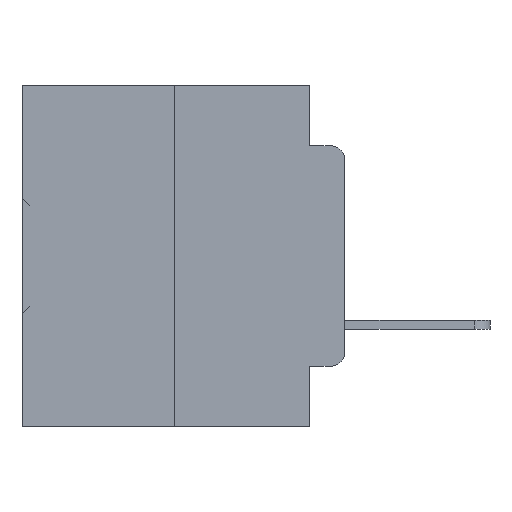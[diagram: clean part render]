
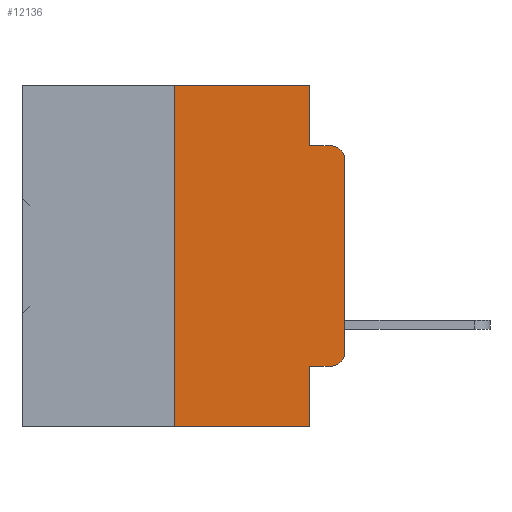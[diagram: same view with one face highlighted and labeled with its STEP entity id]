
A CAD part, left-side view. The second image highlights one B-rep face of the part: STEP entity #12136.
In plain terms, the highlighted planar face has unit normal (-1, 0, 0).
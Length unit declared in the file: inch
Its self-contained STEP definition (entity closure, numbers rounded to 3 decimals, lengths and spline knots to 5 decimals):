
#571 = VECTOR ( 'NONE', #16292, 39.37008 ) ;
#1025 = CARTESIAN_POINT ( 'NONE',  ( 0., 0.051, 0. ) ) ;
#1138 = DIRECTION ( 'NONE',  ( 0., 0., -1. ) ) ;
#1573 = LINE ( 'NONE', #26311, #32571 ) ;
#1580 = LINE ( 'NONE', #21973, #571 ) ;
#2053 = CIRCLE ( 'NONE', #19394, 0.02 ) ;
#2070 = VECTOR ( 'NONE', #13474, 39.37008 ) ;
#2139 = DIRECTION ( 'NONE',  ( 0., -1., 0. ) ) ;
#3630 = PLANE ( 'NONE',  #37530 ) ;
#4343 = EDGE_CURVE ( 'NONE', #12615, #32182, #33869, .T. ) ;
#5000 = CARTESIAN_POINT ( 'NONE',  ( 0., 0.02, -0.1085 ) ) ;
#5078 = VERTEX_POINT ( 'NONE', #11456 ) ;
#5144 = LINE ( 'NONE', #28191, #6150 ) ;
#5808 = CARTESIAN_POINT ( 'NONE',  ( 0., 0.25, 0. ) ) ;
#6150 = VECTOR ( 'NONE', #7257, 39.37008 ) ;
#6776 = CARTESIAN_POINT ( 'NONE',  ( 0., 0., -0.3915 ) ) ;
#6820 = DIRECTION ( 'NONE',  ( 1., 0., 0. ) ) ;
#7229 = VERTEX_POINT ( 'NONE', #32463 ) ;
#7257 = DIRECTION ( 'NONE',  ( 0., 0., -1. ) ) ;
#7376 = VERTEX_POINT ( 'NONE', #6776 ) ;
#7852 = ORIENTED_EDGE ( 'NONE', *, *, #37434, .T. ) ;
#8065 = ORIENTED_EDGE ( 'NONE', *, *, #36766, .T. ) ;
#8166 = DIRECTION ( 'NONE',  ( 0., 0., -1. ) ) ;
#8482 = ORIENTED_EDGE ( 'NONE', *, *, #33053, .F. ) ;
#8788 = ORIENTED_EDGE ( 'NONE', *, *, #32774, .F. ) ;
#9001 = ORIENTED_EDGE ( 'NONE', *, *, #15532, .F. ) ;
#9084 = LINE ( 'NONE', #19105, #24102 ) ;
#9285 = CARTESIAN_POINT ( 'NONE',  ( 0., 0., -0.1085 ) ) ;
#9809 = VECTOR ( 'NONE', #12355, 39.37008 ) ;
#10069 = ORIENTED_EDGE ( 'NONE', *, *, #30841, .F. ) ;
#10225 = ORIENTED_EDGE ( 'NONE', *, *, #4343, .T. ) ;
#11456 = CARTESIAN_POINT ( 'NONE',  ( 0., 0.02, -0.0885 ) ) ;
#11691 = ORIENTED_EDGE ( 'NONE', *, *, #21473, .T. ) ;
#12136 = ADVANCED_FACE ( 'NONE', ( #18305 ), #3630, .F. ) ;
#12290 = ORIENTED_EDGE ( 'NONE', *, *, #24694, .F. ) ;
#12355 = DIRECTION ( 'NONE',  ( 0., 0., 1. ) ) ;
#12615 = VERTEX_POINT ( 'NONE', #27501 ) ;
#13474 = DIRECTION ( 'NONE',  ( 0., -1., 0. ) ) ;
#14044 = CARTESIAN_POINT ( 'NONE',  ( 0., 0.25, 0. ) ) ;
#14267 = DIRECTION ( 'NONE',  ( 0., 0., 1. ) ) ;
#14450 = LINE ( 'NONE', #30665, #20389 ) ;
#15532 = EDGE_CURVE ( 'NONE', #23232, #34252, #14450, .T. ) ;
#16114 = CARTESIAN_POINT ( 'NONE',  ( 0., 0.473, 0. ) ) ;
#16288 = DIRECTION ( 'NONE',  ( 0., -1., 0. ) ) ;
#16292 = DIRECTION ( 'NONE',  ( 0., -1., 0. ) ) ;
#16732 = VERTEX_POINT ( 'NONE', #30584 ) ;
#17167 = LINE ( 'NONE', #37099, #31552 ) ;
#17635 = VERTEX_POINT ( 'NONE', #33755 ) ;
#18305 = FACE_OUTER_BOUND ( 'NONE', #27579, .T. ) ;
#18633 = CIRCLE ( 'NONE', #28339, 0.02 ) ;
#19105 = CARTESIAN_POINT ( 'NONE',  ( 0., 0.051, 0. ) ) ;
#19248 = ORIENTED_EDGE ( 'NONE', *, *, #21204, .T. ) ;
#19394 = AXIS2_PLACEMENT_3D ( 'NONE', #5000, #26105, #8166 ) ;
#19705 = DIRECTION ( 'NONE',  ( -1., 0., 0. ) ) ;
#20389 = VECTOR ( 'NONE', #16288, 39.37008 ) ;
#21204 = EDGE_CURVE ( 'NONE', #7229, #7376, #18633, .T. ) ;
#21473 = EDGE_CURVE ( 'NONE', #17635, #7229, #1573, .T. ) ;
#21973 = CARTESIAN_POINT ( 'NONE',  ( 0., 0.051, -0.0885 ) ) ;
#23232 = VERTEX_POINT ( 'NONE', #14044 ) ;
#24102 = VECTOR ( 'NONE', #33438, 39.37008 ) ;
#24694 = EDGE_CURVE ( 'NONE', #17635, #32182, #9084, .T. ) ;
#25628 = LINE ( 'NONE', #5808, #9809 ) ;
#26105 = DIRECTION ( 'NONE',  ( -1., 0., 0. ) ) ;
#26311 = CARTESIAN_POINT ( 'NONE',  ( 0., 0.051, -0.4115 ) ) ;
#27174 = VERTEX_POINT ( 'NONE', #9285 ) ;
#27501 = CARTESIAN_POINT ( 'NONE',  ( 0., 0.25, -0.5 ) ) ;
#27579 = EDGE_LOOP ( 'NONE', ( #7852, #8065, #8482, #8788, #9001, #10069, #10225, #12290, #11691, #19248 ) ) ;
#27784 = DIRECTION ( 'NONE',  ( 0., 0., -1. ) ) ;
#28191 = CARTESIAN_POINT ( 'NONE',  ( 0., 0.051, 0. ) ) ;
#28339 = AXIS2_PLACEMENT_3D ( 'NONE', #36805, #19705, #1138 ) ;
#30584 = CARTESIAN_POINT ( 'NONE',  ( 0., 0.051, -0.0885 ) ) ;
#30665 = CARTESIAN_POINT ( 'NONE',  ( 0., 0.473, 0. ) ) ;
#30729 = CARTESIAN_POINT ( 'NONE',  ( 0., 0.473, -0.5 ) ) ;
#30841 = EDGE_CURVE ( 'NONE', #12615, #23232, #25628, .T. ) ;
#31552 = VECTOR ( 'NONE', #14267, 39.37008 ) ;
#32182 = VERTEX_POINT ( 'NONE', #36227 ) ;
#32463 = CARTESIAN_POINT ( 'NONE',  ( 0., 0.02, -0.4115 ) ) ;
#32571 = VECTOR ( 'NONE', #2139, 39.37008 ) ;
#32774 = EDGE_CURVE ( 'NONE', #34252, #16732, #5144, .T. ) ;
#33053 = EDGE_CURVE ( 'NONE', #16732, #5078, #1580, .T. ) ;
#33438 = DIRECTION ( 'NONE',  ( 0., 0., -1. ) ) ;
#33755 = CARTESIAN_POINT ( 'NONE',  ( 0., 0.051, -0.4115 ) ) ;
#33869 = LINE ( 'NONE', #30729, #2070 ) ;
#34252 = VERTEX_POINT ( 'NONE', #1025 ) ;
#36227 = CARTESIAN_POINT ( 'NONE',  ( 0., 0.051, -0.5 ) ) ;
#36766 = EDGE_CURVE ( 'NONE', #27174, #5078, #2053, .T. ) ;
#36805 = CARTESIAN_POINT ( 'NONE',  ( 0., 0.02, -0.3915 ) ) ;
#37099 = CARTESIAN_POINT ( 'NONE',  ( 0., 0., 0. ) ) ;
#37434 = EDGE_CURVE ( 'NONE', #7376, #27174, #17167, .T. ) ;
#37530 = AXIS2_PLACEMENT_3D ( 'NONE', #16114, #6820, #27784 ) ;
